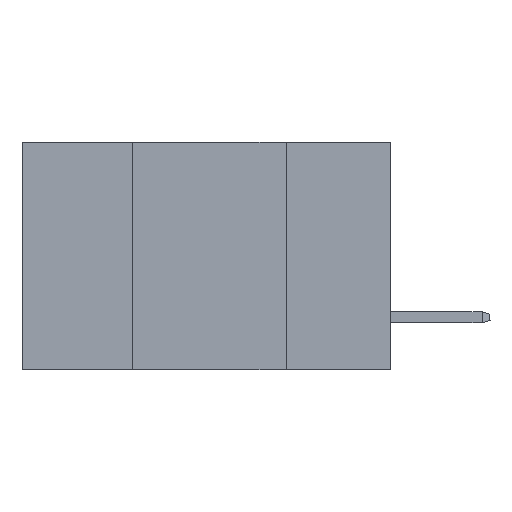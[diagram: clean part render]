
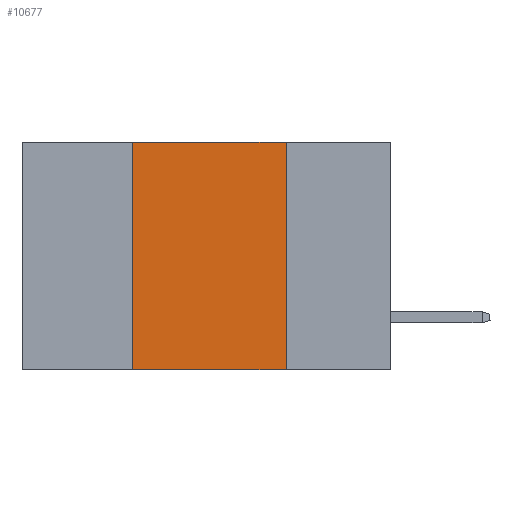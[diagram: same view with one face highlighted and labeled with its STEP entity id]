
A CAD part, left-side view. The second image highlights one B-rep face of the part: STEP entity #10677.
In plain terms, the highlighted planar face has unit normal (-1, 0, 0).
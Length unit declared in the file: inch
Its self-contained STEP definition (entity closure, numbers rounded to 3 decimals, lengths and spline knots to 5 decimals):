
#964 = EDGE_LOOP ( 'NONE', ( #5056, #9712, #2165, #1334 ) ) ;
#1265 = VERTEX_POINT ( 'NONE', #11711 ) ;
#1334 = ORIENTED_EDGE ( 'NONE', *, *, #5705, .T. ) ;
#1399 = AXIS2_PLACEMENT_3D ( 'NONE', #7487, #7710, #3439 ) ;
#1552 = LINE ( 'NONE', #13230, #8375 ) ;
#1947 = CARTESIAN_POINT ( 'NONE',  ( 0., 0.17, 0. ) ) ;
#2165 = ORIENTED_EDGE ( 'NONE', *, *, #11369, .F. ) ;
#2398 = CARTESIAN_POINT ( 'NONE',  ( 0., 0.17, -0.37 ) ) ;
#2438 = DIRECTION ( 'NONE',  ( 0., 0., -1. ) ) ;
#2913 = EDGE_CURVE ( 'NONE', #12153, #12338, #11644, .T. ) ;
#3439 = DIRECTION ( 'NONE',  ( 0., 0., -1. ) ) ;
#3580 = LINE ( 'NONE', #7683, #9901 ) ;
#4822 = VECTOR ( 'NONE', #12702, 39.37008 ) ;
#5056 = ORIENTED_EDGE ( 'NONE', *, *, #8386, .F. ) ;
#5705 = EDGE_CURVE ( 'NONE', #1265, #8253, #12500, .T. ) ;
#5796 = CARTESIAN_POINT ( 'NONE',  ( 0., 0.6, 0. ) ) ;
#7213 = FACE_OUTER_BOUND ( 'NONE', #964, .T. ) ;
#7487 = CARTESIAN_POINT ( 'NONE',  ( 0., 0.6, 0. ) ) ;
#7683 = CARTESIAN_POINT ( 'NONE',  ( 0., 0.42, 0. ) ) ;
#7710 = DIRECTION ( 'NONE',  ( 1., 0., 0. ) ) ;
#8253 = VERTEX_POINT ( 'NONE', #2398 ) ;
#8375 = VECTOR ( 'NONE', #2438, 39.37008 ) ;
#8386 = EDGE_CURVE ( 'NONE', #12338, #8253, #1552, .T. ) ;
#8745 = VECTOR ( 'NONE', #13343, 39.37008 ) ;
#8999 = DIRECTION ( 'NONE',  ( 0., 0., 1. ) ) ;
#9712 = ORIENTED_EDGE ( 'NONE', *, *, #2913, .F. ) ;
#9901 = VECTOR ( 'NONE', #8999, 39.37008 ) ;
#10120 = CARTESIAN_POINT ( 'NONE',  ( 0., 0.42, 0. ) ) ;
#10593 = CARTESIAN_POINT ( 'NONE',  ( 0., 0.6, -0.37 ) ) ;
#10677 = ADVANCED_FACE ( 'NONE', ( #7213 ), #12632, .F. ) ;
#11369 = EDGE_CURVE ( 'NONE', #1265, #12153, #3580, .T. ) ;
#11644 = LINE ( 'NONE', #5796, #8745 ) ;
#11711 = CARTESIAN_POINT ( 'NONE',  ( 0., 0.42, -0.37 ) ) ;
#12153 = VERTEX_POINT ( 'NONE', #10120 ) ;
#12338 = VERTEX_POINT ( 'NONE', #1947 ) ;
#12500 = LINE ( 'NONE', #10593, #4822 ) ;
#12632 = PLANE ( 'NONE',  #1399 ) ;
#12702 = DIRECTION ( 'NONE',  ( 0., -1., 0. ) ) ;
#13230 = CARTESIAN_POINT ( 'NONE',  ( 0., 0.17, 0. ) ) ;
#13343 = DIRECTION ( 'NONE',  ( 0., -1., 0. ) ) ;
